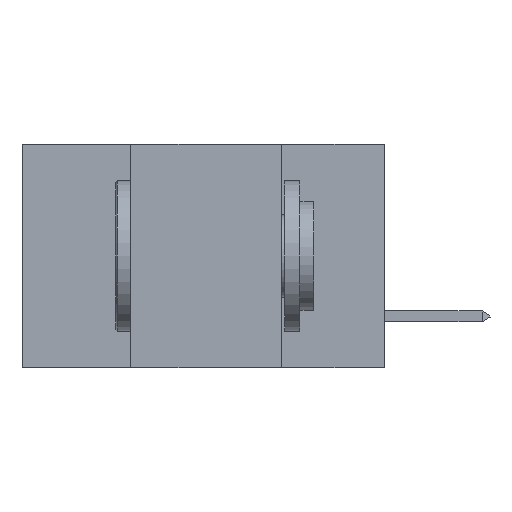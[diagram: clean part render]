
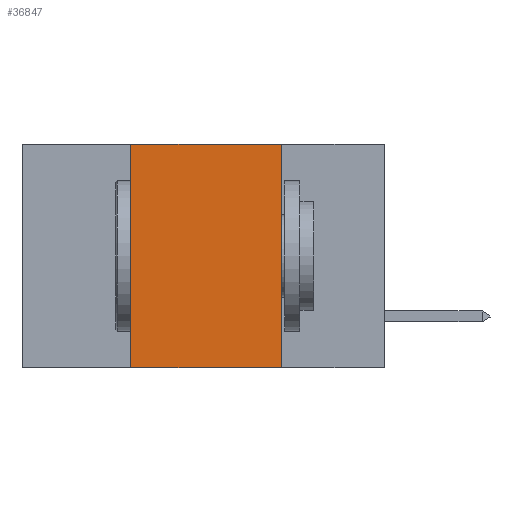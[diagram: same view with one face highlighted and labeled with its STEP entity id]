
A CAD part, left-side view. The second image highlights one B-rep face of the part: STEP entity #36847.
In plain terms, the highlighted planar face has unit normal (-1, 0, 0).
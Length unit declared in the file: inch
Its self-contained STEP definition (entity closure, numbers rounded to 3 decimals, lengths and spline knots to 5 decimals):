
#276 = EDGE_CURVE ( 'NONE', #8709, #30442, #7929, .T. ) ;
#2838 = VECTOR ( 'NONE', #11111, 39.37008 ) ;
#3260 = DIRECTION ( 'NONE',  ( 0., -1., 0. ) ) ;
#4637 = ORIENTED_EDGE ( 'NONE', *, *, #14741, .F. ) ;
#4840 = DIRECTION ( 'NONE',  ( 1., 0., 0. ) ) ;
#5698 = VECTOR ( 'NONE', #10227, 39.37008 ) ;
#6396 = EDGE_CURVE ( 'NONE', #21361, #26934, #21731, .T. ) ;
#7884 = LINE ( 'NONE', #28186, #29455 ) ;
#7929 = LINE ( 'NONE', #28732, #2838 ) ;
#8709 = VERTEX_POINT ( 'NONE', #30706 ) ;
#10227 = DIRECTION ( 'NONE',  ( 0., 0., 1. ) ) ;
#10350 = EDGE_CURVE ( 'NONE', #21361, #30442, #27920, .T. ) ;
#10492 = DIRECTION ( 'NONE',  ( 0., 0., -1. ) ) ;
#11111 = DIRECTION ( 'NONE',  ( 0., 0., -1. ) ) ;
#13511 = AXIS2_PLACEMENT_3D ( 'NONE', #19229, #4840, #10492 ) ;
#14741 = EDGE_CURVE ( 'NONE', #26934, #8709, #7884, .T. ) ;
#16396 = ORIENTED_EDGE ( 'NONE', *, *, #6396, .F. ) ;
#18333 = ORIENTED_EDGE ( 'NONE', *, *, #276, .F. ) ;
#19171 = DIRECTION ( 'NONE',  ( 0., -1., 0. ) ) ;
#19229 = CARTESIAN_POINT ( 'NONE',  ( 0., 0.6, 0. ) ) ;
#19286 = FACE_OUTER_BOUND ( 'NONE', #27027, .T. ) ;
#21361 = VERTEX_POINT ( 'NONE', #29263 ) ;
#21731 = LINE ( 'NONE', #34036, #5698 ) ;
#24861 = CARTESIAN_POINT ( 'NONE',  ( 0., 0.17, -0.37 ) ) ;
#25560 = PLANE ( 'NONE',  #13511 ) ;
#26187 = ORIENTED_EDGE ( 'NONE', *, *, #10350, .T. ) ;
#26934 = VERTEX_POINT ( 'NONE', #36237 ) ;
#27027 = EDGE_LOOP ( 'NONE', ( #18333, #4637, #16396, #26187 ) ) ;
#27920 = LINE ( 'NONE', #35197, #32949 ) ;
#28186 = CARTESIAN_POINT ( 'NONE',  ( 0., 0.6, 0. ) ) ;
#28732 = CARTESIAN_POINT ( 'NONE',  ( 0., 0.17, 0. ) ) ;
#29263 = CARTESIAN_POINT ( 'NONE',  ( 0., 0.42, -0.37 ) ) ;
#29455 = VECTOR ( 'NONE', #19171, 39.37008 ) ;
#30442 = VERTEX_POINT ( 'NONE', #24861 ) ;
#30706 = CARTESIAN_POINT ( 'NONE',  ( 0., 0.17, 0. ) ) ;
#32949 = VECTOR ( 'NONE', #3260, 39.37008 ) ;
#34036 = CARTESIAN_POINT ( 'NONE',  ( 0., 0.42, 0. ) ) ;
#35197 = CARTESIAN_POINT ( 'NONE',  ( 0., 0.6, -0.37 ) ) ;
#36237 = CARTESIAN_POINT ( 'NONE',  ( 0., 0.42, 0. ) ) ;
#36847 = ADVANCED_FACE ( 'NONE', ( #19286 ), #25560, .F. ) ;
